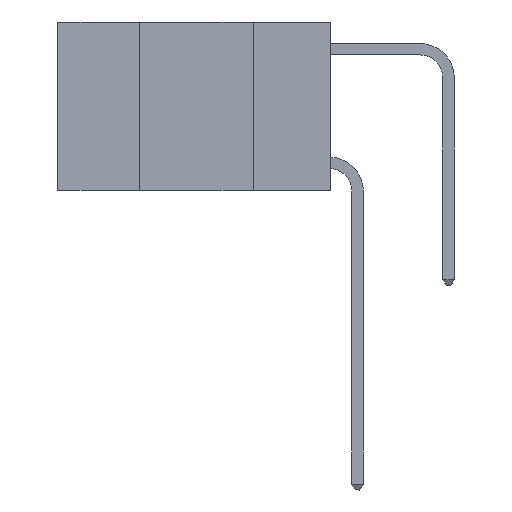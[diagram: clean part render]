
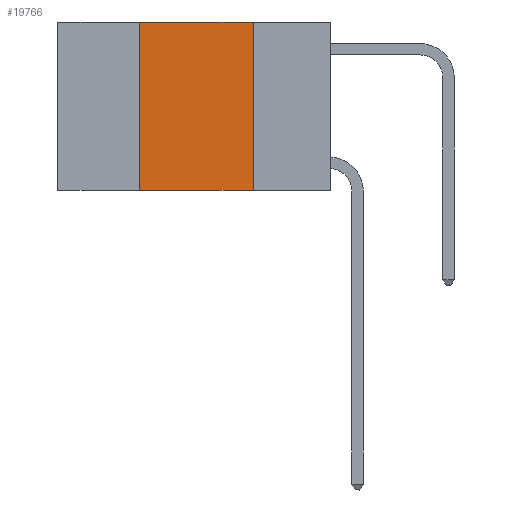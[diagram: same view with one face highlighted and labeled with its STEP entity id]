
A CAD part, left-side view. The second image highlights one B-rep face of the part: STEP entity #19766.
In plain terms, the highlighted planar face has unit normal (-1, 0, 0).
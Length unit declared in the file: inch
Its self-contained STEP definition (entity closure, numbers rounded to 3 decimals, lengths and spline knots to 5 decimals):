
#117 = AXIS2_PLACEMENT_3D ( 'NONE', #10855, #16258, #19638 ) ;
#498 = CARTESIAN_POINT ( 'NONE',  ( 0., 0.6, -0.37 ) ) ;
#686 = CARTESIAN_POINT ( 'NONE',  ( 0., 0.42, 0. ) ) ;
#1409 = DIRECTION ( 'NONE',  ( 0., 0., -1. ) ) ;
#2384 = PLANE ( 'NONE',  #117 ) ;
#2490 = DIRECTION ( 'NONE',  ( 0., 0., 1. ) ) ;
#2592 = VECTOR ( 'NONE', #1409, 39.37008 ) ;
#3111 = VERTEX_POINT ( 'NONE', #21495 ) ;
#3521 = CARTESIAN_POINT ( 'NONE',  ( 0., 0.42, -0.37 ) ) ;
#3587 = ORIENTED_EDGE ( 'NONE', *, *, #8045, .F. ) ;
#5344 = CARTESIAN_POINT ( 'NONE',  ( 0., 0.42, 0. ) ) ;
#5822 = LINE ( 'NONE', #686, #10443 ) ;
#5860 = EDGE_CURVE ( 'NONE', #19076, #3111, #17190, .T. ) ;
#7116 = EDGE_CURVE ( 'NONE', #11932, #19076, #5822, .T. ) ;
#7460 = DIRECTION ( 'NONE',  ( 0., -1., 0. ) ) ;
#7524 = LINE ( 'NONE', #22331, #2592 ) ;
#8045 = EDGE_CURVE ( 'NONE', #3111, #18281, #7524, .T. ) ;
#8856 = ORIENTED_EDGE ( 'NONE', *, *, #7116, .F. ) ;
#9493 = VECTOR ( 'NONE', #7460, 39.37008 ) ;
#9852 = EDGE_CURVE ( 'NONE', #11932, #18281, #20480, .T. ) ;
#10443 = VECTOR ( 'NONE', #2490, 39.37008 ) ;
#10855 = CARTESIAN_POINT ( 'NONE',  ( 0., 0.6, 0. ) ) ;
#11925 = ORIENTED_EDGE ( 'NONE', *, *, #9852, .T. ) ;
#11932 = VERTEX_POINT ( 'NONE', #3521 ) ;
#12784 = DIRECTION ( 'NONE',  ( 0., -1., 0. ) ) ;
#13166 = CARTESIAN_POINT ( 'NONE',  ( 0., 0.17, -0.37 ) ) ;
#13495 = EDGE_LOOP ( 'NONE', ( #3587, #20925, #8856, #11925 ) ) ;
#15913 = FACE_OUTER_BOUND ( 'NONE', #13495, .T. ) ;
#16209 = CARTESIAN_POINT ( 'NONE',  ( 0., 0.6, 0. ) ) ;
#16258 = DIRECTION ( 'NONE',  ( 1., 0., 0. ) ) ;
#17190 = LINE ( 'NONE', #16209, #9493 ) ;
#17820 = VECTOR ( 'NONE', #12784, 39.37008 ) ;
#18281 = VERTEX_POINT ( 'NONE', #13166 ) ;
#19076 = VERTEX_POINT ( 'NONE', #5344 ) ;
#19638 = DIRECTION ( 'NONE',  ( 0., 0., -1. ) ) ;
#19766 = ADVANCED_FACE ( 'NONE', ( #15913 ), #2384, .F. ) ;
#20480 = LINE ( 'NONE', #498, #17820 ) ;
#20925 = ORIENTED_EDGE ( 'NONE', *, *, #5860, .F. ) ;
#21495 = CARTESIAN_POINT ( 'NONE',  ( 0., 0.17, 0. ) ) ;
#22331 = CARTESIAN_POINT ( 'NONE',  ( 0., 0.17, 0. ) ) ;
